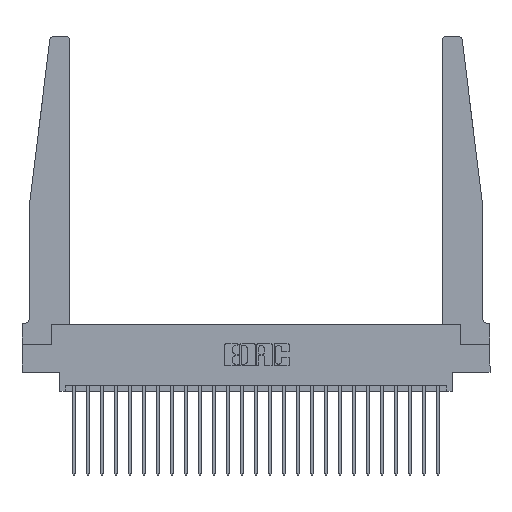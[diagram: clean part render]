
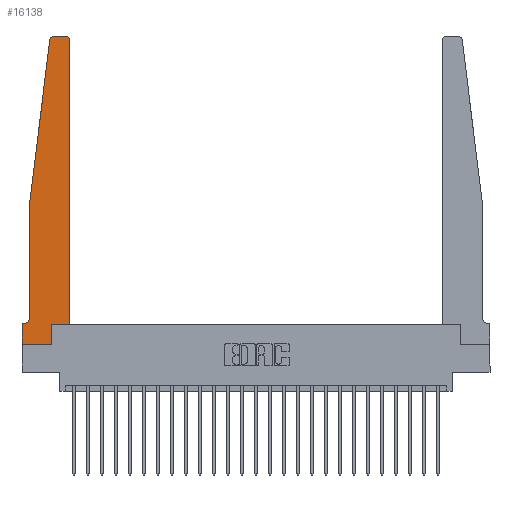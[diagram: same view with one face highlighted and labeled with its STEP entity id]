
A CAD part, top view. The second image highlights one B-rep face of the part: STEP entity #16138.
In plain terms, the highlighted planar face has unit normal (0, 0, 1).
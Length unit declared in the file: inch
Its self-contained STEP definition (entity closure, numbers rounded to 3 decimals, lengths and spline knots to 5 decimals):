
#554 = VECTOR ( 'NONE', #17397, 39.37008 ) ;
#757 = DIRECTION ( 'NONE',  ( 1., 0., 0. ) ) ;
#959 = VERTEX_POINT ( 'NONE', #3264 ) ;
#1173 = FACE_OUTER_BOUND ( 'NONE', #11997, .T. ) ;
#1196 = CIRCLE ( 'NONE', #18565, 0.03 ) ;
#1310 = LINE ( 'NONE', #11192, #7520 ) ;
#1619 = CARTESIAN_POINT ( 'NONE',  ( 0.2605, 0., 0.37 ) ) ;
#1627 = EDGE_CURVE ( 'NONE', #22347, #8812, #17016, .T. ) ;
#1641 = DIRECTION ( 'NONE',  ( 1., 0., 0. ) ) ;
#1667 = ORIENTED_EDGE ( 'NONE', *, *, #15153, .T. ) ;
#2339 = CARTESIAN_POINT ( 'NONE',  ( 0.395, 2.75, 0.37 ) ) ;
#2741 = VERTEX_POINT ( 'NONE', #22077 ) ;
#2842 = EDGE_CURVE ( 'NONE', #2741, #22347, #22247, .T. ) ;
#2992 = EDGE_CURVE ( 'NONE', #3112, #12352, #6090, .T. ) ;
#3107 = EDGE_CURVE ( 'NONE', #12352, #3868, #23204, .T. ) ;
#3112 = VERTEX_POINT ( 'NONE', #21177 ) ;
#3264 = CARTESIAN_POINT ( 'NONE',  ( 0.24675, 2.72367, 0.37 ) ) ;
#3474 = EDGE_CURVE ( 'NONE', #8812, #5361, #17611, .T. ) ;
#3483 = DIRECTION ( 'NONE',  ( 0., 0., 1. ) ) ;
#3603 = DIRECTION ( 'NONE',  ( 1., 0., 0. ) ) ;
#3654 = CARTESIAN_POINT ( 'NONE',  ( 0.2605, 0.18, 0.37 ) ) ;
#3721 = CARTESIAN_POINT ( 'NONE',  ( 0.065, 0.1875, 0.37 ) ) ;
#3868 = VERTEX_POINT ( 'NONE', #8538 ) ;
#4468 = AXIS2_PLACEMENT_3D ( 'NONE', #18160, #16275, #6649 ) ;
#4880 = AXIS2_PLACEMENT_3D ( 'NONE', #19520, #7652, #6003 ) ;
#5331 = EDGE_CURVE ( 'NONE', #3868, #959, #1196, .T. ) ;
#5357 = ORIENTED_EDGE ( 'NONE', *, *, #3107, .T. ) ;
#5361 = VERTEX_POINT ( 'NONE', #10181 ) ;
#5372 = VECTOR ( 'NONE', #23141, 39.37008 ) ;
#5738 = ORIENTED_EDGE ( 'NONE', *, *, #5331, .T. ) ;
#6003 = DIRECTION ( 'NONE',  ( 1., 0., 0. ) ) ;
#6090 = CIRCLE ( 'NONE', #4880, 0.03 ) ;
#6489 = CARTESIAN_POINT ( 'NONE',  ( 0.015, 0.1875, 0.37 ) ) ;
#6649 = DIRECTION ( 'NONE',  ( -1., 0., 0. ) ) ;
#6881 = EDGE_CURVE ( 'NONE', #14630, #3112, #1310, .T. ) ;
#7044 = EDGE_CURVE ( 'NONE', #8038, #13786, #19735, .T. ) ;
#7075 = VECTOR ( 'NONE', #17242, 39.37008 ) ;
#7520 = VECTOR ( 'NONE', #21026, 39.37008 ) ;
#7652 = DIRECTION ( 'NONE',  ( 0., 0., 1. ) ) ;
#8038 = VERTEX_POINT ( 'NONE', #1619 ) ;
#8538 = CARTESIAN_POINT ( 'NONE',  ( 0.27653, 2.75, 0.37 ) ) ;
#8565 = EDGE_CURVE ( 'NONE', #959, #16879, #13624, .T. ) ;
#8582 = ORIENTED_EDGE ( 'NONE', *, *, #15151, .T. ) ;
#8760 = PLANE ( 'NONE',  #23981 ) ;
#8812 = VERTEX_POINT ( 'NONE', #12457 ) ;
#9357 = CARTESIAN_POINT ( 'NONE',  ( 0.065, 1.25, 0.37 ) ) ;
#9556 = CARTESIAN_POINT ( 'NONE',  ( 0.25, 2.75, 0.37 ) ) ;
#9859 = LINE ( 'NONE', #15450, #5372 ) ;
#9981 = VECTOR ( 'NONE', #17621, 39.37008 ) ;
#10181 = CARTESIAN_POINT ( 'NONE',  ( 0., 0., 0.37 ) ) ;
#10234 = VECTOR ( 'NONE', #757, 39.37008 ) ;
#10518 = CARTESIAN_POINT ( 'NONE',  ( 0., 0., 0.37 ) ) ;
#10552 = DIRECTION ( 'NONE',  ( 0., 0., 1. ) ) ;
#10928 = ORIENTED_EDGE ( 'NONE', *, *, #6881, .T. ) ;
#11192 = CARTESIAN_POINT ( 'NONE',  ( 0.425, 0.18, 0.37 ) ) ;
#11347 = CARTESIAN_POINT ( 'NONE',  ( 0.065, 1.25, 0.37 ) ) ;
#11965 = ORIENTED_EDGE ( 'NONE', *, *, #8565, .T. ) ;
#11997 = EDGE_LOOP ( 'NONE', ( #5357, #5738, #11965, #8582, #13183, #18035, #16320, #15278, #15090, #1667, #10928, #22777 ) ) ;
#12352 = VERTEX_POINT ( 'NONE', #2339 ) ;
#12457 = CARTESIAN_POINT ( 'NONE',  ( 0., 0.1875, 0.37 ) ) ;
#13183 = ORIENTED_EDGE ( 'NONE', *, *, #2842, .T. ) ;
#13624 = LINE ( 'NONE', #11347, #14834 ) ;
#13667 = CARTESIAN_POINT ( 'NONE',  ( 0.425, 0.18, 0.37 ) ) ;
#13786 = VERTEX_POINT ( 'NONE', #3654 ) ;
#14354 = CARTESIAN_POINT ( 'NONE',  ( 0., 0.1875, 0.37 ) ) ;
#14630 = VERTEX_POINT ( 'NONE', #23166 ) ;
#14834 = VECTOR ( 'NONE', #19526, 39.37008 ) ;
#14845 = EDGE_CURVE ( 'NONE', #5361, #8038, #17971, .T. ) ;
#15090 = ORIENTED_EDGE ( 'NONE', *, *, #7044, .T. ) ;
#15151 = EDGE_CURVE ( 'NONE', #16879, #2741, #9859, .T. ) ;
#15153 = EDGE_CURVE ( 'NONE', #13786, #14630, #15323, .T. ) ;
#15278 = ORIENTED_EDGE ( 'NONE', *, *, #14845, .T. ) ;
#15323 = LINE ( 'NONE', #13667, #18296 ) ;
#15450 = CARTESIAN_POINT ( 'NONE',  ( 0.065, 1.25, 0.37 ) ) ;
#16138 = ADVANCED_FACE ( 'NONE', ( #1173 ), #8760, .T. ) ;
#16275 = DIRECTION ( 'NONE',  ( 0., 0., -1. ) ) ;
#16320 = ORIENTED_EDGE ( 'NONE', *, *, #3474, .T. ) ;
#16879 = VERTEX_POINT ( 'NONE', #9357 ) ;
#17016 = LINE ( 'NONE', #3721, #554 ) ;
#17242 = DIRECTION ( 'NONE',  ( 0., -1., 0. ) ) ;
#17397 = DIRECTION ( 'NONE',  ( -1., 0., 0. ) ) ;
#17493 = CARTESIAN_POINT ( 'NONE',  ( 0., 0., 0.37 ) ) ;
#17611 = LINE ( 'NONE', #17493, #7075 ) ;
#17621 = DIRECTION ( 'NONE',  ( 0., 1., 0. ) ) ;
#17971 = LINE ( 'NONE', #10518, #10234 ) ;
#18035 = ORIENTED_EDGE ( 'NONE', *, *, #1627, .T. ) ;
#18160 = CARTESIAN_POINT ( 'NONE',  ( 0.015, 0.2375, 0.37 ) ) ;
#18296 = VECTOR ( 'NONE', #1641, 39.37008 ) ;
#18501 = DIRECTION ( 'NONE',  ( 1., 0., 0. ) ) ;
#18565 = AXIS2_PLACEMENT_3D ( 'NONE', #18669, #3483, #3603 ) ;
#18669 = CARTESIAN_POINT ( 'NONE',  ( 0.27653, 2.72, 0.37 ) ) ;
#19019 = VECTOR ( 'NONE', #19040, 39.37008 ) ;
#19040 = DIRECTION ( 'NONE',  ( -1., 0., 0. ) ) ;
#19520 = CARTESIAN_POINT ( 'NONE',  ( 0.395, 2.72, 0.37 ) ) ;
#19526 = DIRECTION ( 'NONE',  ( -0.122, -0.992, 0. ) ) ;
#19735 = LINE ( 'NONE', #21527, #9981 ) ;
#21026 = DIRECTION ( 'NONE',  ( 0., 1., 0. ) ) ;
#21177 = CARTESIAN_POINT ( 'NONE',  ( 0.425, 2.72, 0.37 ) ) ;
#21527 = CARTESIAN_POINT ( 'NONE',  ( 0.2605, 0.18, 0.37 ) ) ;
#22077 = CARTESIAN_POINT ( 'NONE',  ( 0.065, 0.2375, 0.37 ) ) ;
#22247 = CIRCLE ( 'NONE', #4468, 0.05 ) ;
#22347 = VERTEX_POINT ( 'NONE', #6489 ) ;
#22777 = ORIENTED_EDGE ( 'NONE', *, *, #2992, .T. ) ;
#23141 = DIRECTION ( 'NONE',  ( 0., -1., 0. ) ) ;
#23166 = CARTESIAN_POINT ( 'NONE',  ( 0.425, 0.18, 0.37 ) ) ;
#23204 = LINE ( 'NONE', #9556, #19019 ) ;
#23981 = AXIS2_PLACEMENT_3D ( 'NONE', #14354, #10552, #18501 ) ;
